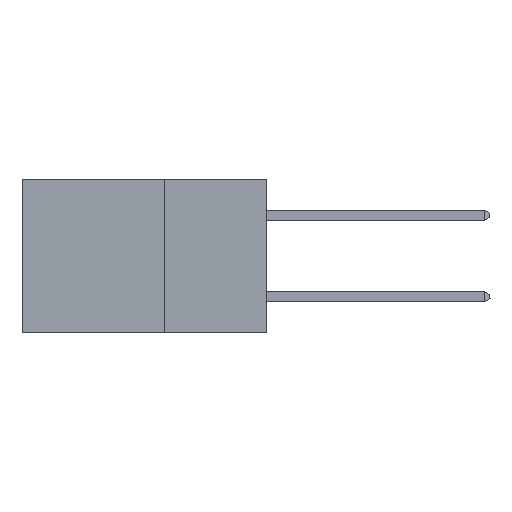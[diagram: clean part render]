
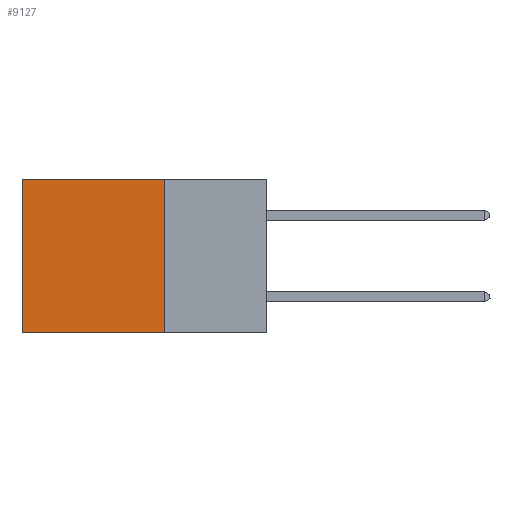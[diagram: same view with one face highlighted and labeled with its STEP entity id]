
A CAD part, left-side view. The second image highlights one B-rep face of the part: STEP entity #9127.
In plain terms, the highlighted planar face has unit normal (-1, 0, 0).
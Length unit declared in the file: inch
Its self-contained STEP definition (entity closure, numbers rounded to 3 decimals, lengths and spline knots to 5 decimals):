
#714 = LINE ( 'NONE', #8653, #8079 ) ;
#984 = CARTESIAN_POINT ( 'NONE',  ( 0.2875, 0.25, -0.375 ) ) ;
#1586 = CARTESIAN_POINT ( 'NONE',  ( 0.2875, 0.25, -0.375 ) ) ;
#1938 = CARTESIAN_POINT ( 'NONE',  ( 0.2875, 0.6, -0.375 ) ) ;
#2639 = DIRECTION ( 'NONE',  ( 0., 1., 0. ) ) ;
#2913 = VERTEX_POINT ( 'NONE', #3134 ) ;
#3134 = CARTESIAN_POINT ( 'NONE',  ( 0.2875, 0.25, 0. ) ) ;
#3394 = LINE ( 'NONE', #12959, #4815 ) ;
#3402 = DIRECTION ( 'NONE',  ( 0., 0., -1. ) ) ;
#4109 = CARTESIAN_POINT ( 'NONE',  ( 0.2875, 0.6, -0.375 ) ) ;
#4603 = DIRECTION ( 'NONE',  ( 0., 0., -1. ) ) ;
#4709 = VECTOR ( 'NONE', #4603, 39.37008 ) ;
#4815 = VECTOR ( 'NONE', #2639, 39.37008 ) ;
#4996 = FACE_OUTER_BOUND ( 'NONE', #14843, .T. ) ;
#5413 = ORIENTED_EDGE ( 'NONE', *, *, #12097, .T. ) ;
#7494 = EDGE_CURVE ( 'NONE', #2913, #9390, #714, .T. ) ;
#7524 = PLANE ( 'NONE',  #12940 ) ;
#8079 = VECTOR ( 'NONE', #3402, 39.37008 ) ;
#8556 = LINE ( 'NONE', #1586, #12840 ) ;
#8653 = CARTESIAN_POINT ( 'NONE',  ( 0.2875, 0.25, -0.375 ) ) ;
#9127 = ADVANCED_FACE ( 'NONE', ( #4996 ), #7524, .F. ) ;
#9390 = VERTEX_POINT ( 'NONE', #984 ) ;
#9644 = VERTEX_POINT ( 'NONE', #11022 ) ;
#10142 = ORIENTED_EDGE ( 'NONE', *, *, #16500, .T. ) ;
#10650 = DIRECTION ( 'NONE',  ( 0., 1., 0. ) ) ;
#11022 = CARTESIAN_POINT ( 'NONE',  ( 0.2875, 0.6, 0. ) ) ;
#11802 = ORIENTED_EDGE ( 'NONE', *, *, #16585, .F. ) ;
#12097 = EDGE_CURVE ( 'NONE', #9644, #14002, #13025, .T. ) ;
#12840 = VECTOR ( 'NONE', #10650, 39.37008 ) ;
#12940 = AXIS2_PLACEMENT_3D ( 'NONE', #16642, #15159, #16528 ) ;
#12959 = CARTESIAN_POINT ( 'NONE',  ( 0.2875, 0.25, 0. ) ) ;
#13025 = LINE ( 'NONE', #1938, #4709 ) ;
#14002 = VERTEX_POINT ( 'NONE', #4109 ) ;
#14790 = ORIENTED_EDGE ( 'NONE', *, *, #7494, .F. ) ;
#14843 = EDGE_LOOP ( 'NONE', ( #5413, #11802, #14790, #10142 ) ) ;
#15159 = DIRECTION ( 'NONE',  ( 1., 0., 0. ) ) ;
#16500 = EDGE_CURVE ( 'NONE', #2913, #9644, #3394, .T. ) ;
#16528 = DIRECTION ( 'NONE',  ( 0., 0., -1. ) ) ;
#16585 = EDGE_CURVE ( 'NONE', #9390, #14002, #8556, .T. ) ;
#16642 = CARTESIAN_POINT ( 'NONE',  ( 0.2875, 0.25, -0.375 ) ) ;
